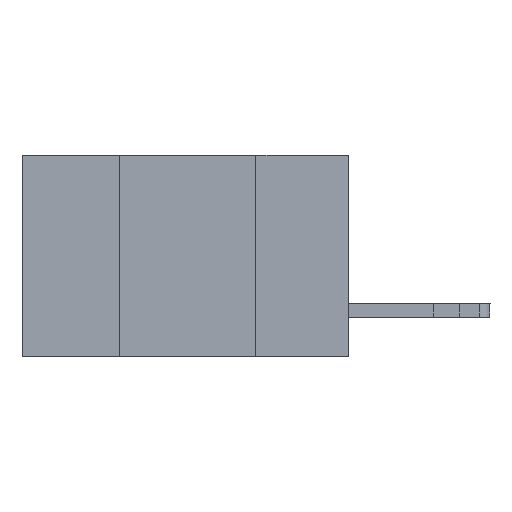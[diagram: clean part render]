
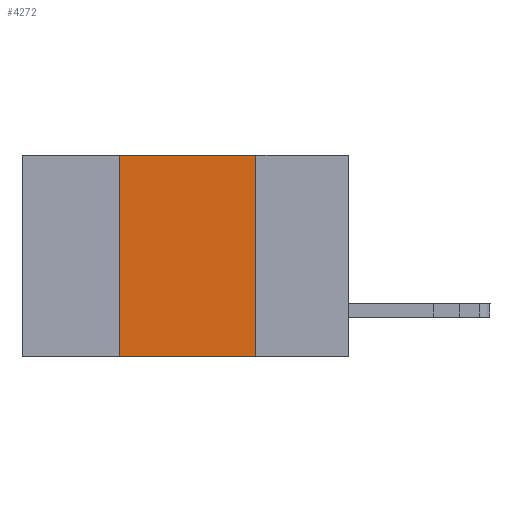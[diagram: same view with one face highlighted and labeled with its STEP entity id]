
A CAD part, left-side view. The second image highlights one B-rep face of the part: STEP entity #4272.
In plain terms, the highlighted planar face has unit normal (-1, 0, 0).
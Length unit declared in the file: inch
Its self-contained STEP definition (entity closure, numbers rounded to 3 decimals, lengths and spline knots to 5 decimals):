
#7 = FACE_OUTER_BOUND ( 'NONE', #13017, .T. ) ;
#301 = ORIENTED_EDGE ( 'NONE', *, *, #11027, .F. ) ;
#378 = LINE ( 'NONE', #6652, #3401 ) ;
#417 = LINE ( 'NONE', #5862, #6809 ) ;
#988 = ORIENTED_EDGE ( 'NONE', *, *, #2188, .F. ) ;
#1213 = CARTESIAN_POINT ( 'NONE',  ( 0., 0.17, -0.37 ) ) ;
#2188 = EDGE_CURVE ( 'NONE', #5376, #5022, #14011, .T. ) ;
#3385 = CARTESIAN_POINT ( 'NONE',  ( 0., 0.42, 0. ) ) ;
#3396 = ORIENTED_EDGE ( 'NONE', *, *, #5125, .F. ) ;
#3401 = VECTOR ( 'NONE', #10581, 39.37008 ) ;
#4272 = ADVANCED_FACE ( 'NONE', ( #7 ), #13132, .F. ) ;
#4504 = VERTEX_POINT ( 'NONE', #1213 ) ;
#5022 = VERTEX_POINT ( 'NONE', #13048 ) ;
#5125 = EDGE_CURVE ( 'NONE', #5022, #4504, #378, .T. ) ;
#5153 = ORIENTED_EDGE ( 'NONE', *, *, #15078, .T. ) ;
#5306 = CARTESIAN_POINT ( 'NONE',  ( 0., 0.42, 0. ) ) ;
#5376 = VERTEX_POINT ( 'NONE', #3385 ) ;
#5550 = DIRECTION ( 'NONE',  ( 1., 0., 0. ) ) ;
#5862 = CARTESIAN_POINT ( 'NONE',  ( 0., 0.6, -0.37 ) ) ;
#6326 = CARTESIAN_POINT ( 'NONE',  ( 0., 0.42, -0.37 ) ) ;
#6652 = CARTESIAN_POINT ( 'NONE',  ( 0., 0.17, 0. ) ) ;
#6809 = VECTOR ( 'NONE', #13455, 39.37008 ) ;
#6908 = VERTEX_POINT ( 'NONE', #6326 ) ;
#9438 = VECTOR ( 'NONE', #10304, 39.37008 ) ;
#9452 = DIRECTION ( 'NONE',  ( 0., 0., -1. ) ) ;
#10304 = DIRECTION ( 'NONE',  ( 0., 0., 1. ) ) ;
#10581 = DIRECTION ( 'NONE',  ( 0., 0., -1. ) ) ;
#10674 = CARTESIAN_POINT ( 'NONE',  ( 0., 0.6, 0. ) ) ;
#11027 = EDGE_CURVE ( 'NONE', #6908, #5376, #14217, .T. ) ;
#12638 = VECTOR ( 'NONE', #13316, 39.37008 ) ;
#13017 = EDGE_LOOP ( 'NONE', ( #3396, #988, #301, #5153 ) ) ;
#13048 = CARTESIAN_POINT ( 'NONE',  ( 0., 0.17, 0. ) ) ;
#13132 = PLANE ( 'NONE',  #15186 ) ;
#13316 = DIRECTION ( 'NONE',  ( 0., -1., 0. ) ) ;
#13455 = DIRECTION ( 'NONE',  ( 0., -1., 0. ) ) ;
#14011 = LINE ( 'NONE', #15556, #12638 ) ;
#14217 = LINE ( 'NONE', #5306, #9438 ) ;
#15078 = EDGE_CURVE ( 'NONE', #6908, #4504, #417, .T. ) ;
#15186 = AXIS2_PLACEMENT_3D ( 'NONE', #10674, #5550, #9452 ) ;
#15556 = CARTESIAN_POINT ( 'NONE',  ( 0., 0.6, 0. ) ) ;
